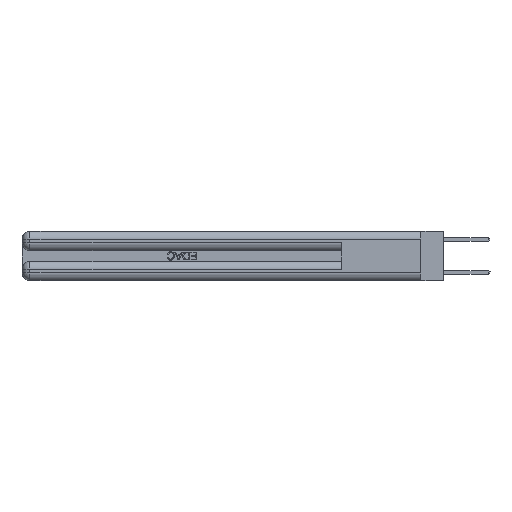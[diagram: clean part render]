
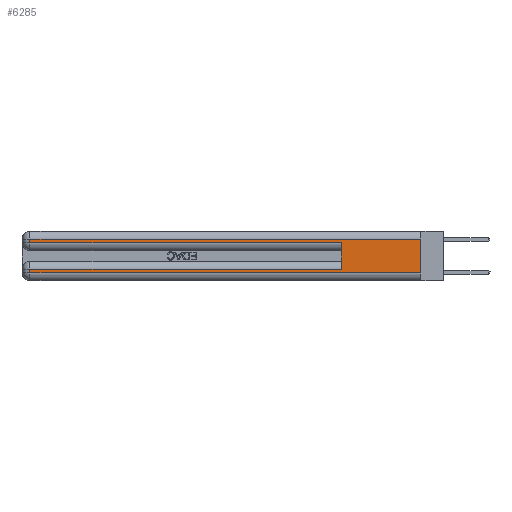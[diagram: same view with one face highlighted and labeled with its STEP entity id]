
A CAD part, left-side view. The second image highlights one B-rep face of the part: STEP entity #6285.
In plain terms, the highlighted planar face has unit normal (-1, 0, 0).
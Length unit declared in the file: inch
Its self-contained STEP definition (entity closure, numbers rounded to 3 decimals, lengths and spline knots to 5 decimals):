
#635 = VERTEX_POINT ( 'NONE', #20994 ) ;
#821 = DIRECTION ( 'NONE',  ( 0., 1., 0. ) ) ;
#905 = VECTOR ( 'NONE', #5570, 39.37008 ) ;
#1700 = ORIENTED_EDGE ( 'NONE', *, *, #10676, .F. ) ;
#2150 = EDGE_CURVE ( 'NONE', #18617, #2665, #17552, .T. ) ;
#2665 = VERTEX_POINT ( 'NONE', #10365 ) ;
#2895 = VECTOR ( 'NONE', #6194, 39.37008 ) ;
#2969 = CARTESIAN_POINT ( 'NONE',  ( 0., 0., 0.285 ) ) ;
#3132 = CARTESIAN_POINT ( 'NONE',  ( 0., 2.94, 0.285 ) ) ;
#3489 = VERTEX_POINT ( 'NONE', #10861 ) ;
#4099 = EDGE_CURVE ( 'NONE', #7316, #30815, #30524, .T. ) ;
#4189 = VECTOR ( 'NONE', #8812, 39.37008 ) ;
#5422 = VECTOR ( 'NONE', #22362, 39.37008 ) ;
#5570 = DIRECTION ( 'NONE',  ( 0., 0., -1. ) ) ;
#5874 = LINE ( 'NONE', #11413, #11639 ) ;
#6194 = DIRECTION ( 'NONE',  ( 0., -1., 0. ) ) ;
#6228 = CARTESIAN_POINT ( 'NONE',  ( 0., 0.6, 0.145 ) ) ;
#6285 = ADVANCED_FACE ( 'NONE', ( #11887 ), #29770, .F. ) ;
#7068 = LINE ( 'NONE', #2969, #19142 ) ;
#7112 = EDGE_CURVE ( 'NONE', #18617, #26798, #11466, .T. ) ;
#7316 = VERTEX_POINT ( 'NONE', #26400 ) ;
#7970 = ORIENTED_EDGE ( 'NONE', *, *, #23787, .T. ) ;
#7993 = CARTESIAN_POINT ( 'NONE',  ( 0., 0., 0.085 ) ) ;
#8671 = LINE ( 'NONE', #11018, #2895 ) ;
#8698 = ORIENTED_EDGE ( 'NONE', *, *, #13627, .T. ) ;
#8812 = DIRECTION ( 'NONE',  ( 0., 0., 1. ) ) ;
#10365 = CARTESIAN_POINT ( 'NONE',  ( 0., 2.94, 0.085 ) ) ;
#10386 = EDGE_CURVE ( 'NONE', #25024, #26798, #7068, .T. ) ;
#10611 = CARTESIAN_POINT ( 'NONE',  ( 0., 0., 0.31 ) ) ;
#10676 = EDGE_CURVE ( 'NONE', #7316, #3489, #5874, .T. ) ;
#10861 = CARTESIAN_POINT ( 'NONE',  ( 0., 0., 0.06 ) ) ;
#11018 = CARTESIAN_POINT ( 'NONE',  ( 0., 0., 0.06 ) ) ;
#11413 = CARTESIAN_POINT ( 'NONE',  ( 0., 0., 0.37 ) ) ;
#11466 = LINE ( 'NONE', #6228, #4189 ) ;
#11486 = VECTOR ( 'NONE', #821, 39.37008 ) ;
#11639 = VECTOR ( 'NONE', #25719, 39.37008 ) ;
#11887 = FACE_OUTER_BOUND ( 'NONE', #29269, .T. ) ;
#12199 = VECTOR ( 'NONE', #28399, 39.37008 ) ;
#12651 = CARTESIAN_POINT ( 'NONE',  ( 0., 0.6, 0.085 ) ) ;
#13627 = EDGE_CURVE ( 'NONE', #30815, #25024, #25860, .T. ) ;
#15510 = CARTESIAN_POINT ( 'NONE',  ( 0., 0., 0.37 ) ) ;
#16524 = CARTESIAN_POINT ( 'NONE',  ( 0., 2.94, 0.37 ) ) ;
#17552 = LINE ( 'NONE', #7993, #5422 ) ;
#17889 = DIRECTION ( 'NONE',  ( 0., 0., -1. ) ) ;
#18617 = VERTEX_POINT ( 'NONE', #12651 ) ;
#19007 = AXIS2_PLACEMENT_3D ( 'NONE', #15510, #24966, #17889 ) ;
#19142 = VECTOR ( 'NONE', #24570, 39.37008 ) ;
#20027 = CARTESIAN_POINT ( 'NONE',  ( 0., 2.94, 0.37 ) ) ;
#20994 = CARTESIAN_POINT ( 'NONE',  ( 0., 2.94, 0.06 ) ) ;
#21782 = ORIENTED_EDGE ( 'NONE', *, *, #4099, .T. ) ;
#22362 = DIRECTION ( 'NONE',  ( 0., 1., 0. ) ) ;
#22436 = CARTESIAN_POINT ( 'NONE',  ( 0., 0.6, 0.285 ) ) ;
#23328 = CARTESIAN_POINT ( 'NONE',  ( 0., 2.94, 0.31 ) ) ;
#23383 = LINE ( 'NONE', #16524, #12199 ) ;
#23787 = EDGE_CURVE ( 'NONE', #635, #3489, #8671, .T. ) ;
#24570 = DIRECTION ( 'NONE',  ( 0., -1., 0. ) ) ;
#24711 = ORIENTED_EDGE ( 'NONE', *, *, #7112, .F. ) ;
#24966 = DIRECTION ( 'NONE',  ( 1., 0., 0. ) ) ;
#25024 = VERTEX_POINT ( 'NONE', #3132 ) ;
#25719 = DIRECTION ( 'NONE',  ( 0., 0., -1. ) ) ;
#25860 = LINE ( 'NONE', #20027, #905 ) ;
#26400 = CARTESIAN_POINT ( 'NONE',  ( 0., 0., 0.31 ) ) ;
#26798 = VERTEX_POINT ( 'NONE', #22436 ) ;
#28399 = DIRECTION ( 'NONE',  ( 0., 0., -1. ) ) ;
#29269 = EDGE_LOOP ( 'NONE', ( #1700, #21782, #8698, #30659, #24711, #29956, #31169, #7970 ) ) ;
#29770 = PLANE ( 'NONE',  #19007 ) ;
#29956 = ORIENTED_EDGE ( 'NONE', *, *, #2150, .T. ) ;
#30177 = EDGE_CURVE ( 'NONE', #2665, #635, #23383, .T. ) ;
#30524 = LINE ( 'NONE', #10611, #11486 ) ;
#30659 = ORIENTED_EDGE ( 'NONE', *, *, #10386, .T. ) ;
#30815 = VERTEX_POINT ( 'NONE', #23328 ) ;
#31169 = ORIENTED_EDGE ( 'NONE', *, *, #30177, .T. ) ;
